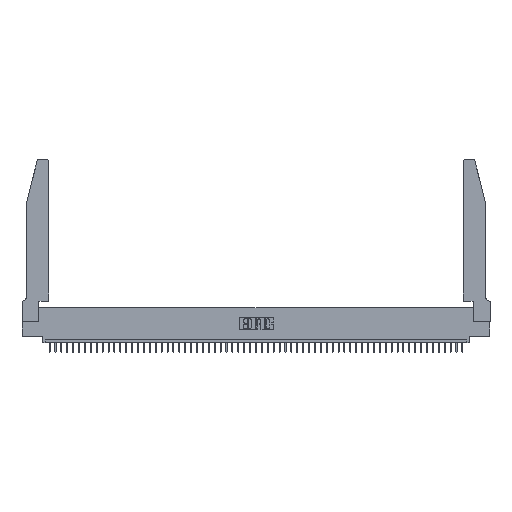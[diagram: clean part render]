
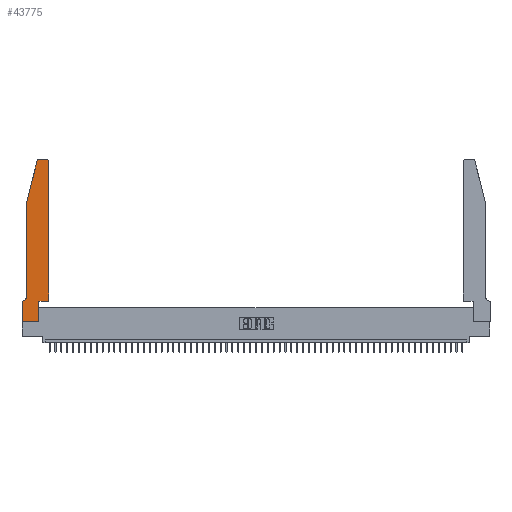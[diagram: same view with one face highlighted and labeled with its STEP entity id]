
A CAD part, top view. The second image highlights one B-rep face of the part: STEP entity #43775.
In plain terms, the highlighted planar face has unit normal (0, 0, 1).
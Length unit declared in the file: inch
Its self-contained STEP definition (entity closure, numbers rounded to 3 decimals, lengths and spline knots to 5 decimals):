
#788 = LINE ( 'NONE', #53538, #27252 ) ;
#2736 = EDGE_CURVE ( 'NONE', #43804, #34807, #46887, .T. ) ;
#2877 = ORIENTED_EDGE ( 'NONE', *, *, #10781, .T. ) ;
#4483 = DIRECTION ( 'NONE',  ( 0., 0., 1. ) ) ;
#4844 = CARTESIAN_POINT ( 'NONE',  ( 0.0755, 0.35, 0.37 ) ) ;
#5120 = EDGE_CURVE ( 'NONE', #49425, #8246, #36930, .T. ) ;
#5724 = LINE ( 'NONE', #27803, #38123 ) ;
#6414 = DIRECTION ( 'NONE',  ( -0.239, -0.971, 0. ) ) ;
#7665 = FACE_OUTER_BOUND ( 'NONE', #25864, .T. ) ;
#7667 = VERTEX_POINT ( 'NONE', #44868 ) ;
#7910 = EDGE_CURVE ( 'NONE', #23452, #27375, #788, .T. ) ;
#8246 = VERTEX_POINT ( 'NONE', #40228 ) ;
#8506 = CARTESIAN_POINT ( 'NONE',  ( 0., 0., 0.37 ) ) ;
#10246 = DIRECTION ( 'NONE',  ( 0., 1., 0. ) ) ;
#10411 = ORIENTED_EDGE ( 'NONE', *, *, #34214, .T. ) ;
#10767 = DIRECTION ( 'NONE',  ( -1., 0., 0. ) ) ;
#10781 = EDGE_CURVE ( 'NONE', #7667, #39756, #42646, .T. ) ;
#10946 = VECTOR ( 'NONE', #25646, 39.37008 ) ;
#12313 = VECTOR ( 'NONE', #10246, 39.37008 ) ;
#12574 = AXIS2_PLACEMENT_3D ( 'NONE', #12596, #4483, #17153 ) ;
#12596 = CARTESIAN_POINT ( 'NONE',  ( 0.4205, 2.72, 0.37 ) ) ;
#12730 = LINE ( 'NONE', #53150, #17922 ) ;
#13031 = CIRCLE ( 'NONE', #40133, 0.07 ) ;
#14046 = CARTESIAN_POINT ( 'NONE',  ( 0.2865, 0.35, 0.37 ) ) ;
#14413 = ORIENTED_EDGE ( 'NONE', *, *, #40621, .T. ) ;
#15577 = DIRECTION ( 'NONE',  ( -1., 0., 0. ) ) ;
#15706 = VERTEX_POINT ( 'NONE', #32197 ) ;
#17077 = ORIENTED_EDGE ( 'NONE', *, *, #38103, .T. ) ;
#17153 = DIRECTION ( 'NONE',  ( 1., 0., 0. ) ) ;
#17894 = DIRECTION ( 'NONE',  ( 1., 0., 0. ) ) ;
#17922 = VECTOR ( 'NONE', #6414, 39.37008 ) ;
#18713 = CARTESIAN_POINT ( 'NONE',  ( 0.284, 2.72, 0.37 ) ) ;
#18953 = AXIS2_PLACEMENT_3D ( 'NONE', #41123, #19945, #44931 ) ;
#19945 = DIRECTION ( 'NONE',  ( 0., 0., 1. ) ) ;
#20947 = ORIENTED_EDGE ( 'NONE', *, *, #42744, .T. ) ;
#21116 = CARTESIAN_POINT ( 'NONE',  ( 0., 0.35, 0.37 ) ) ;
#22532 = EDGE_CURVE ( 'NONE', #27375, #7667, #13031, .T. ) ;
#23452 = VERTEX_POINT ( 'NONE', #31650 ) ;
#23484 = LINE ( 'NONE', #8506, #10946 ) ;
#23515 = DIRECTION ( 'NONE',  ( -1., 0., 0. ) ) ;
#23732 = VECTOR ( 'NONE', #40305, 39.37008 ) ;
#25176 = ORIENTED_EDGE ( 'NONE', *, *, #7910, .T. ) ;
#25248 = CARTESIAN_POINT ( 'NONE',  ( 0.2865, 0., 0.37 ) ) ;
#25646 = DIRECTION ( 'NONE',  ( 0., -1., 0. ) ) ;
#25864 = EDGE_LOOP ( 'NONE', ( #52318, #20947, #17077, #25176, #38205, #2877, #10411, #34071, #26230, #14413, #26480, #47222 ) ) ;
#26230 = ORIENTED_EDGE ( 'NONE', *, *, #5120, .T. ) ;
#26471 = VERTEX_POINT ( 'NONE', #43743 ) ;
#26480 = ORIENTED_EDGE ( 'NONE', *, *, #52008, .T. ) ;
#27252 = VECTOR ( 'NONE', #44279, 39.37008 ) ;
#27375 = VERTEX_POINT ( 'NONE', #43136 ) ;
#27803 = CARTESIAN_POINT ( 'NONE',  ( 0.4505, 0.35, 0.37 ) ) ;
#28139 = CARTESIAN_POINT ( 'NONE',  ( 0.0055, 0.42, 0.37 ) ) ;
#29263 = VECTOR ( 'NONE', #17894, 39.37008 ) ;
#29453 = CIRCLE ( 'NONE', #40873, 0.03 ) ;
#29487 = EDGE_CURVE ( 'NONE', #15706, #43804, #48897, .T. ) ;
#31650 = CARTESIAN_POINT ( 'NONE',  ( 0.0755, 2., 0.37 ) ) ;
#32197 = CARTESIAN_POINT ( 'NONE',  ( 0.4505, 2.72, 0.37 ) ) ;
#32987 = VERTEX_POINT ( 'NONE', #48700 ) ;
#34071 = ORIENTED_EDGE ( 'NONE', *, *, #36192, .T. ) ;
#34214 = EDGE_CURVE ( 'NONE', #39756, #32987, #23484, .T. ) ;
#34807 = VERTEX_POINT ( 'NONE', #38054 ) ;
#35766 = VECTOR ( 'NONE', #23515, 39.37008 ) ;
#36192 = EDGE_CURVE ( 'NONE', #32987, #49425, #49567, .T. ) ;
#36580 = DIRECTION ( 'NONE',  ( 0., 0., -1. ) ) ;
#36848 = DIRECTION ( 'NONE',  ( 1., 0., 0. ) ) ;
#36930 = LINE ( 'NONE', #14046, #23732 ) ;
#38054 = CARTESIAN_POINT ( 'NONE',  ( 0.284, 2.75, 0.37 ) ) ;
#38103 = EDGE_CURVE ( 'NONE', #26471, #23452, #12730, .T. ) ;
#38123 = VECTOR ( 'NONE', #36848, 39.37008 ) ;
#38205 = ORIENTED_EDGE ( 'NONE', *, *, #22532, .T. ) ;
#38527 = VERTEX_POINT ( 'NONE', #53676 ) ;
#39756 = VERTEX_POINT ( 'NONE', #21116 ) ;
#40133 = AXIS2_PLACEMENT_3D ( 'NONE', #28139, #36580, #15577 ) ;
#40228 = CARTESIAN_POINT ( 'NONE',  ( 0.2865, 0.35, 0.37 ) ) ;
#40305 = DIRECTION ( 'NONE',  ( 0., 1., 0. ) ) ;
#40621 = EDGE_CURVE ( 'NONE', #8246, #38527, #5724, .T. ) ;
#40873 = AXIS2_PLACEMENT_3D ( 'NONE', #18713, #47711, #48098 ) ;
#41123 = CARTESIAN_POINT ( 'NONE',  ( 0., 0.35, 0.37 ) ) ;
#42646 = LINE ( 'NONE', #4844, #49937 ) ;
#42744 = EDGE_CURVE ( 'NONE', #34807, #26471, #29453, .T. ) ;
#43136 = CARTESIAN_POINT ( 'NONE',  ( 0.0755, 0.42, 0.37 ) ) ;
#43743 = CARTESIAN_POINT ( 'NONE',  ( 0.25487, 2.72718, 0.37 ) ) ;
#43775 = ADVANCED_FACE ( 'NONE', ( #7665 ), #45133, .T. ) ;
#43804 = VERTEX_POINT ( 'NONE', #45314 ) ;
#44279 = DIRECTION ( 'NONE',  ( 0., -1., 0. ) ) ;
#44868 = CARTESIAN_POINT ( 'NONE',  ( 0.0055, 0.35, 0.37 ) ) ;
#44931 = DIRECTION ( 'NONE',  ( 1., 0., 0. ) ) ;
#45133 = PLANE ( 'NONE',  #18953 ) ;
#45314 = CARTESIAN_POINT ( 'NONE',  ( 0.4205, 2.75, 0.37 ) ) ;
#46887 = LINE ( 'NONE', #52686, #35766 ) ;
#47222 = ORIENTED_EDGE ( 'NONE', *, *, #29487, .T. ) ;
#47711 = DIRECTION ( 'NONE',  ( 0., 0., 1. ) ) ;
#47719 = CARTESIAN_POINT ( 'NONE',  ( 0.4505, 0.35, 0.37 ) ) ;
#48098 = DIRECTION ( 'NONE',  ( 1., 0., 0. ) ) ;
#48389 = LINE ( 'NONE', #47719, #12313 ) ;
#48700 = CARTESIAN_POINT ( 'NONE',  ( 0., 0., 0.37 ) ) ;
#48897 = CIRCLE ( 'NONE', #12574, 0.03 ) ;
#49425 = VERTEX_POINT ( 'NONE', #25248 ) ;
#49567 = LINE ( 'NONE', #52066, #29263 ) ;
#49937 = VECTOR ( 'NONE', #10767, 39.37008 ) ;
#52008 = EDGE_CURVE ( 'NONE', #38527, #15706, #48389, .T. ) ;
#52066 = CARTESIAN_POINT ( 'NONE',  ( 0., 0., 0.37 ) ) ;
#52318 = ORIENTED_EDGE ( 'NONE', *, *, #2736, .T. ) ;
#52686 = CARTESIAN_POINT ( 'NONE',  ( 0.2605, 2.75, 0.37 ) ) ;
#53150 = CARTESIAN_POINT ( 'NONE',  ( 0.0755, 2., 0.37 ) ) ;
#53538 = CARTESIAN_POINT ( 'NONE',  ( 0.0755, 2., 0.37 ) ) ;
#53676 = CARTESIAN_POINT ( 'NONE',  ( 0.4505, 0.35, 0.37 ) ) ;
